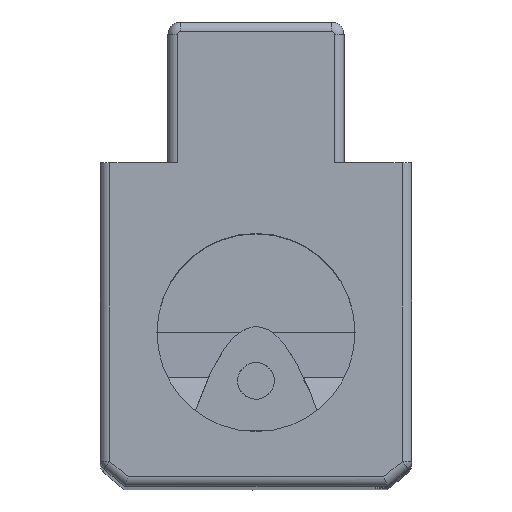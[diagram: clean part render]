
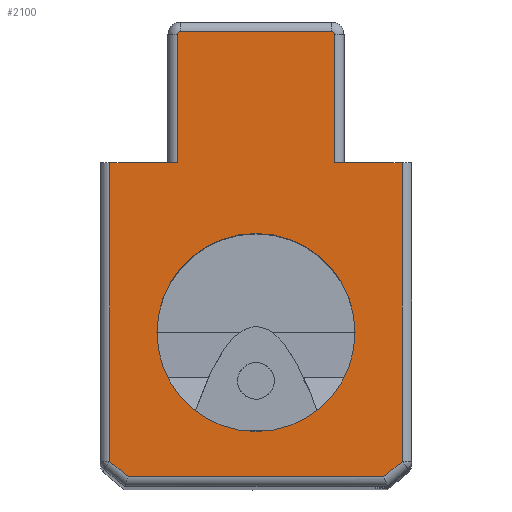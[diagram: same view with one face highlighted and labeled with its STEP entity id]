
A CAD part, top view. The second image highlights one B-rep face of the part: STEP entity #2100.
In plain terms, the highlighted planar face has unit normal (0, 0, 1).
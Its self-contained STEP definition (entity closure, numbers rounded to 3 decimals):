
#3 = LINE ( 'NONE', #592, #274 ) ;
#158 = VERTEX_POINT ( 'NONE', #3214 ) ;
#220 = VECTOR ( 'NONE', #5429, 1000. ) ;
#256 = DIRECTION ( 'NONE',  ( -1., 0., 0. ) ) ;
#257 = CARTESIAN_POINT ( 'NONE',  ( -6.4, 23.75, 0. ) ) ;
#274 = VECTOR ( 'NONE', #432, 1000. ) ;
#375 = DIRECTION ( 'NONE',  ( -0.766, 0.643, 0. ) ) ;
#387 = CARTESIAN_POINT ( 'NONE',  ( 11.95, -11.199, 0. ) ) ;
#392 = EDGE_CURVE ( 'NONE', #2811, #574, #3, .T. ) ;
#432 = DIRECTION ( 'NONE',  ( 1., 0., 0. ) ) ;
#445 = CARTESIAN_POINT ( 'NONE',  ( -6.4, 13.25, 0. ) ) ;
#447 = LINE ( 'NONE', #1704, #1818 ) ;
#448 = VERTEX_POINT ( 'NONE', #257 ) ;
#574 = VERTEX_POINT ( 'NONE', #445 ) ;
#592 = CARTESIAN_POINT ( 'NONE',  ( -12.75, 13.25, 0. ) ) ;
#615 = EDGE_CURVE ( 'NONE', #2900, #2811, #447, .T. ) ;
#691 = DIRECTION ( 'NONE',  ( -1., 0., 0. ) ) ;
#851 = ORIENTED_EDGE ( 'NONE', *, *, #2279, .T. ) ;
#881 = CARTESIAN_POINT ( 'NONE',  ( 0., -0.65, 0. ) ) ;
#912 = LINE ( 'NONE', #1000, #3436 ) ;
#950 = CARTESIAN_POINT ( 'NONE',  ( 6.4, 23.75, 0. ) ) ;
#1000 = CARTESIAN_POINT ( 'NONE',  ( -10.459, -12.45, 0. ) ) ;
#1015 = CARTESIAN_POINT ( 'NONE',  ( 11.95, 0., 0. ) ) ;
#1019 = LINE ( 'NONE', #1015, #3773 ) ;
#1024 = CARTESIAN_POINT ( 'NONE',  ( -11.95, -11.199, 0. ) ) ;
#1037 = ORIENTED_EDGE ( 'NONE', *, *, #1597, .T. ) ;
#1165 = DIRECTION ( 'NONE',  ( 0., 0., 1. ) ) ;
#1184 = CARTESIAN_POINT ( 'NONE',  ( -6.4, 13.25, 0. ) ) ;
#1253 = EDGE_LOOP ( 'NONE', ( #5158, #2648, #3185, #3808, #5454, #3145, #5373, #2067, #2371, #5151, #1037, #4130 ) ) ;
#1273 = EDGE_LOOP ( 'NONE', ( #2169, #851 ) ) ;
#1310 = EDGE_CURVE ( 'NONE', #1942, #2887, #1858, .T. ) ;
#1328 = CARTESIAN_POINT ( 'NONE',  ( 6.2, 23.75, 0. ) ) ;
#1369 = CARTESIAN_POINT ( 'NONE',  ( -6.2, 23.95, 0. ) ) ;
#1428 = LINE ( 'NONE', #5330, #1835 ) ;
#1439 = LINE ( 'NONE', #1902, #1463 ) ;
#1463 = VECTOR ( 'NONE', #1536, 1000. ) ;
#1536 = DIRECTION ( 'NONE',  ( 0., 1., 0. ) ) ;
#1597 = EDGE_CURVE ( 'NONE', #158, #2642, #2761, .T. ) ;
#1606 = CARTESIAN_POINT ( 'NONE',  ( 10.459, -12.45, 0. ) ) ;
#1704 = CARTESIAN_POINT ( 'NONE',  ( -11.95, 0., 0. ) ) ;
#1818 = VECTOR ( 'NONE', #3025, 1000. ) ;
#1835 = VECTOR ( 'NONE', #3553, 1000. ) ;
#1858 = CIRCLE ( 'NONE', #3625, 8.1 ) ;
#1884 = DIRECTION ( 'NONE',  ( -1., 0., 0. ) ) ;
#1902 = CARTESIAN_POINT ( 'NONE',  ( 6.4, 0., 0. ) ) ;
#1942 = VERTEX_POINT ( 'NONE', #4705 ) ;
#2059 = AXIS2_PLACEMENT_3D ( 'NONE', #4353, #1165, #691 ) ;
#2067 = ORIENTED_EDGE ( 'NONE', *, *, #3781, .F. ) ;
#2100 = ADVANCED_FACE ( 'NONE', ( #4262, #2588 ), #3895, .F. ) ;
#2169 = ORIENTED_EDGE ( 'NONE', *, *, #1310, .T. ) ;
#2279 = EDGE_CURVE ( 'NONE', #2887, #1942, #2733, .T. ) ;
#2371 = ORIENTED_EDGE ( 'NONE', *, *, #3520, .T. ) ;
#2396 = VECTOR ( 'NONE', #3007, 1000. ) ;
#2452 = CARTESIAN_POINT ( 'NONE',  ( -11.95, 13.25, 0. ) ) ;
#2481 = EDGE_CURVE ( 'NONE', #2998, #158, #4642, .T. ) ;
#2588 = FACE_OUTER_BOUND ( 'NONE', #1253, .T. ) ;
#2615 = LINE ( 'NONE', #1184, #4080 ) ;
#2629 = AXIS2_PLACEMENT_3D ( 'NONE', #4613, #2675, #3795 ) ;
#2642 = VERTEX_POINT ( 'NONE', #1369 ) ;
#2648 = ORIENTED_EDGE ( 'NONE', *, *, #392, .F. ) ;
#2675 = DIRECTION ( 'NONE',  ( 0., 0., -1. ) ) ;
#2733 = CIRCLE ( 'NONE', #3936, 8.1 ) ;
#2761 = LINE ( 'NONE', #3705, #2899 ) ;
#2811 = VERTEX_POINT ( 'NONE', #2452 ) ;
#2848 = AXIS2_PLACEMENT_3D ( 'NONE', #1328, #4812, #1884 ) ;
#2887 = VERTEX_POINT ( 'NONE', #4029 ) ;
#2899 = VECTOR ( 'NONE', #4342, 1000. ) ;
#2900 = VERTEX_POINT ( 'NONE', #1024 ) ;
#2998 = VERTEX_POINT ( 'NONE', #950 ) ;
#3007 = DIRECTION ( 'NONE',  ( 1., 0., 0. ) ) ;
#3021 = CIRCLE ( 'NONE', #2059, 0.2 ) ;
#3025 = DIRECTION ( 'NONE',  ( 0., 1., 0. ) ) ;
#3092 = LINE ( 'NONE', #5386, #2396 ) ;
#3145 = ORIENTED_EDGE ( 'NONE', *, *, #3524, .F. ) ;
#3149 = VERTEX_POINT ( 'NONE', #3791 ) ;
#3185 = ORIENTED_EDGE ( 'NONE', *, *, #615, .F. ) ;
#3214 = CARTESIAN_POINT ( 'NONE',  ( 6.2, 23.95, 0. ) ) ;
#3296 = VERTEX_POINT ( 'NONE', #1606 ) ;
#3395 = CARTESIAN_POINT ( 'NONE',  ( -10.459, -12.45, 0. ) ) ;
#3436 = VECTOR ( 'NONE', #375, 1000. ) ;
#3520 = EDGE_CURVE ( 'NONE', #5023, #2998, #1439, .T. ) ;
#3524 = EDGE_CURVE ( 'NONE', #3149, #3296, #5004, .T. ) ;
#3553 = DIRECTION ( 'NONE',  ( -1., 0., 0. ) ) ;
#3625 = AXIS2_PLACEMENT_3D ( 'NONE', #881, #4331, #256 ) ;
#3628 = EDGE_CURVE ( 'NONE', #448, #574, #2615, .T. ) ;
#3705 = CARTESIAN_POINT ( 'NONE',  ( -6.2, 23.95, 0. ) ) ;
#3773 = VECTOR ( 'NONE', #5440, 1000. ) ;
#3781 = EDGE_CURVE ( 'NONE', #5023, #4369, #3092, .T. ) ;
#3791 = CARTESIAN_POINT ( 'NONE',  ( 11.95, -11.199, 0. ) ) ;
#3795 = DIRECTION ( 'NONE',  ( -1., 0., 0. ) ) ;
#3808 = ORIENTED_EDGE ( 'NONE', *, *, #4381, .F. ) ;
#3895 = PLANE ( 'NONE',  #2629 ) ;
#3936 = AXIS2_PLACEMENT_3D ( 'NONE', #4009, #4917, #5163 ) ;
#4009 = CARTESIAN_POINT ( 'NONE',  ( 0., -0.65, 0. ) ) ;
#4029 = CARTESIAN_POINT ( 'NONE',  ( -8.1, -0.65, 0. ) ) ;
#4080 = VECTOR ( 'NONE', #5180, 1000. ) ;
#4130 = ORIENTED_EDGE ( 'NONE', *, *, #4155, .T. ) ;
#4155 = EDGE_CURVE ( 'NONE', #2642, #448, #3021, .T. ) ;
#4241 = EDGE_CURVE ( 'NONE', #3296, #5212, #1428, .T. ) ;
#4262 = FACE_BOUND ( 'NONE', #1273, .T. ) ;
#4331 = DIRECTION ( 'NONE',  ( 0., 0., -1. ) ) ;
#4342 = DIRECTION ( 'NONE',  ( -1., 0., 0. ) ) ;
#4353 = CARTESIAN_POINT ( 'NONE',  ( -6.2, 23.75, 0. ) ) ;
#4369 = VERTEX_POINT ( 'NONE', #4899 ) ;
#4381 = EDGE_CURVE ( 'NONE', #5212, #2900, #912, .T. ) ;
#4546 = CARTESIAN_POINT ( 'NONE',  ( 6.4, 13.25, 0. ) ) ;
#4613 = CARTESIAN_POINT ( 'NONE',  ( 0., 0., 0. ) ) ;
#4642 = CIRCLE ( 'NONE', #2848, 0.2 ) ;
#4705 = CARTESIAN_POINT ( 'NONE',  ( 8.1, -0.65, 0. ) ) ;
#4812 = DIRECTION ( 'NONE',  ( 0., 0., 1. ) ) ;
#4899 = CARTESIAN_POINT ( 'NONE',  ( 11.95, 13.25, 0. ) ) ;
#4917 = DIRECTION ( 'NONE',  ( 0., 0., -1. ) ) ;
#5004 = LINE ( 'NONE', #387, #220 ) ;
#5023 = VERTEX_POINT ( 'NONE', #4546 ) ;
#5151 = ORIENTED_EDGE ( 'NONE', *, *, #2481, .T. ) ;
#5158 = ORIENTED_EDGE ( 'NONE', *, *, #3628, .T. ) ;
#5163 = DIRECTION ( 'NONE',  ( -1., 0., 0. ) ) ;
#5180 = DIRECTION ( 'NONE',  ( 0., -1., 0. ) ) ;
#5194 = EDGE_CURVE ( 'NONE', #4369, #3149, #1019, .T. ) ;
#5212 = VERTEX_POINT ( 'NONE', #3395 ) ;
#5330 = CARTESIAN_POINT ( 'NONE',  ( 0., -12.45, 0. ) ) ;
#5373 = ORIENTED_EDGE ( 'NONE', *, *, #5194, .F. ) ;
#5386 = CARTESIAN_POINT ( 'NONE',  ( -12.75, 13.25, 0. ) ) ;
#5429 = DIRECTION ( 'NONE',  ( -0.766, -0.643, 0. ) ) ;
#5440 = DIRECTION ( 'NONE',  ( 0., -1., 0. ) ) ;
#5454 = ORIENTED_EDGE ( 'NONE', *, *, #4241, .F. ) ;
